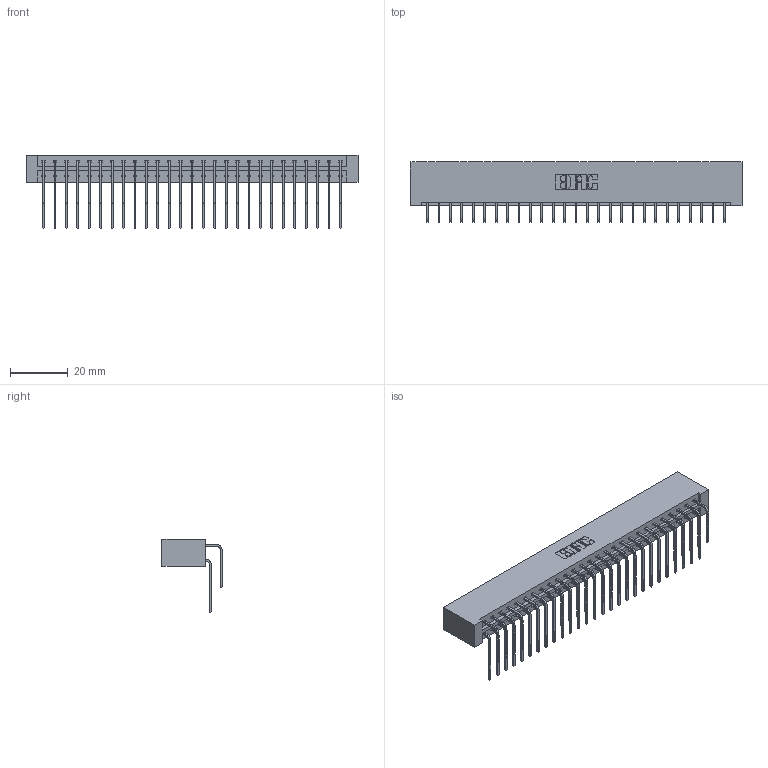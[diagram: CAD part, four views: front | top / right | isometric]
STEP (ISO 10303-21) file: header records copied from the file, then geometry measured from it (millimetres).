
FILE_DESCRIPTION (( 'STEP AP203' ), '1' );
FILE_NAME ('833-054-559-201.STEP', '2020-06-04T21:43:40', ( '' ), ( '' ), 'SwSTEP 2.0', 'SolidWorks 2020', '' );
FILE_SCHEMA (( 'CONFIG_CONTROL_DESIGN' ));
Length unit declared in the file: inch
Products named in the file (4): 345-292-001_558 559 Tail - 1; 833 Part_Lugless; 833-054-559-201; 345-292-001_559 Tail - 2
Assembly tree (55 placements, depth 2):
  833-054-559-201
    833 Part_Lugless
    345-292-001_558 559 Tail - 1  x27
    345-292-001_559 Tail - 2  x27
Bounding box: 115.24 x 20.9 x 25.53 mm (x, y, z)
Volume: 12568.8 mm3; surface area: 16274.3 mm2
Topology: 55 solids, 55 shells, 3022 faces, 8981 edges, 5914 vertices
Faces by surface type: plane 2118, cylinder 904
Entity records: 20817 total; most frequent: CARTESIAN_POINT 3517, ORIENTED_EDGE 3402, DIRECTION 3005, EDGE_CURVE 1701, VECTOR 1541, LINE 1541, VERTEX_POINT 1130, AXIS2_PLACEMENT_3D 732
